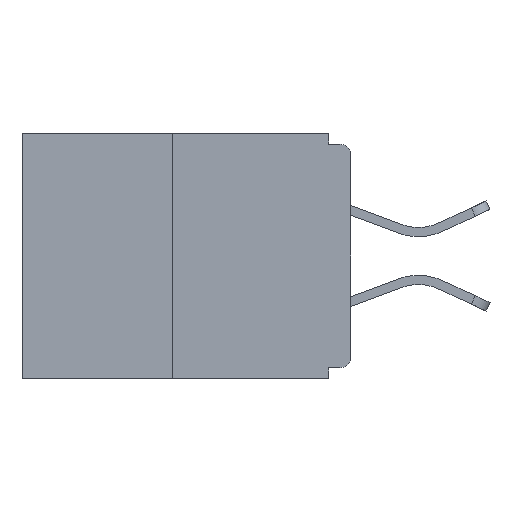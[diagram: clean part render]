
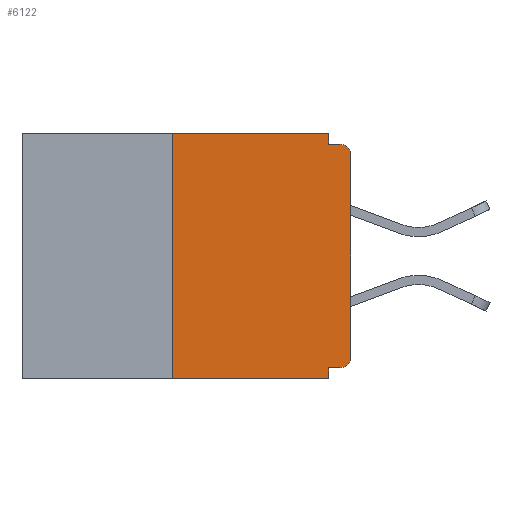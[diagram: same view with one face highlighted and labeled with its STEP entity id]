
A CAD part, left-side view. The second image highlights one B-rep face of the part: STEP entity #6122.
In plain terms, the highlighted planar face has unit normal (-1, 0, 0).
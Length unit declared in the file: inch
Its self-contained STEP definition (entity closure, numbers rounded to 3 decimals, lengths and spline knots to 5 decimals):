
#109 = CARTESIAN_POINT ( 'NONE',  ( 0., 0.015, -0.03 ) ) ;
#169 = ORIENTED_EDGE ( 'NONE', *, *, #7103, .T. ) ;
#346 = AXIS2_PLACEMENT_3D ( 'NONE', #14062, #10802, #5309 ) ;
#379 = VECTOR ( 'NONE', #10592, 39.37008 ) ;
#384 = EDGE_CURVE ( 'NONE', #3862, #9873, #11531, .T. ) ;
#671 = CARTESIAN_POINT ( 'NONE',  ( 0., 0.031, -0.343 ) ) ;
#859 = DIRECTION ( 'NONE',  ( 0., -1., 0. ) ) ;
#1123 = ORIENTED_EDGE ( 'NONE', *, *, #3468, .T. ) ;
#1216 = VERTEX_POINT ( 'NONE', #6062 ) ;
#1294 = CARTESIAN_POINT ( 'NONE',  ( 0., 0.46, -0.343 ) ) ;
#1317 = VERTEX_POINT ( 'NONE', #8545 ) ;
#1413 = VECTOR ( 'NONE', #2914, 39.37008 ) ;
#1504 = VERTEX_POINT ( 'NONE', #9048 ) ;
#2130 = ORIENTED_EDGE ( 'NONE', *, *, #5068, .F. ) ;
#2186 = CARTESIAN_POINT ( 'NONE',  ( 0., 0., -0.03 ) ) ;
#2205 = VERTEX_POINT ( 'NONE', #10170 ) ;
#2299 = CARTESIAN_POINT ( 'NONE',  ( 0., 0.031, 0. ) ) ;
#2351 = CARTESIAN_POINT ( 'NONE',  ( 0., 0.015, -0.015 ) ) ;
#2426 = LINE ( 'NONE', #5913, #7983 ) ;
#2914 = DIRECTION ( 'NONE',  ( 0., -1., 0. ) ) ;
#3018 = VERTEX_POINT ( 'NONE', #6176 ) ;
#3104 = CARTESIAN_POINT ( 'NONE',  ( 0., 0.46, 0. ) ) ;
#3373 = CARTESIAN_POINT ( 'NONE',  ( 0., 0.46, 0. ) ) ;
#3398 = DIRECTION ( 'NONE',  ( -1., 0., 0. ) ) ;
#3468 = EDGE_CURVE ( 'NONE', #1216, #13208, #2426, .T. ) ;
#3528 = VECTOR ( 'NONE', #7657, 39.37008 ) ;
#3664 = LINE ( 'NONE', #6067, #379 ) ;
#3862 = VERTEX_POINT ( 'NONE', #13517 ) ;
#3998 = DIRECTION ( 'NONE',  ( 0., 0., -1. ) ) ;
#4060 = ORIENTED_EDGE ( 'NONE', *, *, #7364, .T. ) ;
#4066 = ORIENTED_EDGE ( 'NONE', *, *, #5152, .F. ) ;
#4101 = CIRCLE ( 'NONE', #4241, 0.015 ) ;
#4130 = ORIENTED_EDGE ( 'NONE', *, *, #4430, .F. ) ;
#4160 = LINE ( 'NONE', #671, #8690 ) ;
#4241 = AXIS2_PLACEMENT_3D ( 'NONE', #109, #3398, #11175 ) ;
#4396 = DIRECTION ( 'NONE',  ( 1., 0., 0. ) ) ;
#4430 = EDGE_CURVE ( 'NONE', #1504, #2205, #3664, .T. ) ;
#5024 = ORIENTED_EDGE ( 'NONE', *, *, #384, .F. ) ;
#5068 = EDGE_CURVE ( 'NONE', #7882, #3018, #14091, .T. ) ;
#5152 = EDGE_CURVE ( 'NONE', #3018, #1317, #4160, .T. ) ;
#5309 = DIRECTION ( 'NONE',  ( 0., 0., -1. ) ) ;
#5508 = DIRECTION ( 'NONE',  ( 0., 0., -1. ) ) ;
#5756 = DIRECTION ( 'NONE',  ( 0., -1., 0. ) ) ;
#5913 = CARTESIAN_POINT ( 'NONE',  ( 0., 0., 0. ) ) ;
#6062 = CARTESIAN_POINT ( 'NONE',  ( 0., 0., -0.313 ) ) ;
#6067 = CARTESIAN_POINT ( 'NONE',  ( 0., 0.25, 0. ) ) ;
#6122 = ADVANCED_FACE ( 'NONE', ( #12318 ), #6695, .F. ) ;
#6176 = CARTESIAN_POINT ( 'NONE',  ( 0., 0.031, -0.328 ) ) ;
#6589 = CARTESIAN_POINT ( 'NONE',  ( 0., 0.015, -0.328 ) ) ;
#6695 = PLANE ( 'NONE',  #8813 ) ;
#7103 = EDGE_CURVE ( 'NONE', #7882, #1216, #7399, .T. ) ;
#7364 = EDGE_CURVE ( 'NONE', #13208, #9873, #4101, .T. ) ;
#7399 = CIRCLE ( 'NONE', #346, 0.015 ) ;
#7434 = CARTESIAN_POINT ( 'NONE',  ( 0., 0., -0.015 ) ) ;
#7574 = ORIENTED_EDGE ( 'NONE', *, *, #11496, .T. ) ;
#7657 = DIRECTION ( 'NONE',  ( 0., 0., -1. ) ) ;
#7812 = VECTOR ( 'NONE', #8400, 39.37008 ) ;
#7882 = VERTEX_POINT ( 'NONE', #6589 ) ;
#7983 = VECTOR ( 'NONE', #8113, 39.37008 ) ;
#7995 = VECTOR ( 'NONE', #5756, 39.37008 ) ;
#8113 = DIRECTION ( 'NONE',  ( 0., 0., 1. ) ) ;
#8400 = DIRECTION ( 'NONE',  ( 0., 1., 0. ) ) ;
#8540 = EDGE_CURVE ( 'NONE', #12053, #3862, #11366, .T. ) ;
#8545 = CARTESIAN_POINT ( 'NONE',  ( 0., 0.031, -0.343 ) ) ;
#8690 = VECTOR ( 'NONE', #3998, 39.37008 ) ;
#8813 = AXIS2_PLACEMENT_3D ( 'NONE', #3373, #4396, #5508 ) ;
#9048 = CARTESIAN_POINT ( 'NONE',  ( 0., 0.25, -0.343 ) ) ;
#9873 = VERTEX_POINT ( 'NONE', #2351 ) ;
#10170 = CARTESIAN_POINT ( 'NONE',  ( 0., 0.25, 0. ) ) ;
#10174 = ORIENTED_EDGE ( 'NONE', *, *, #8540, .F. ) ;
#10241 = EDGE_CURVE ( 'NONE', #2205, #12053, #11855, .T. ) ;
#10592 = DIRECTION ( 'NONE',  ( 0., 0., 1. ) ) ;
#10802 = DIRECTION ( 'NONE',  ( -1., 0., 0. ) ) ;
#10960 = LINE ( 'NONE', #1294, #7995 ) ;
#11175 = DIRECTION ( 'NONE',  ( 0., 0., -1. ) ) ;
#11192 = VECTOR ( 'NONE', #859, 39.37008 ) ;
#11366 = LINE ( 'NONE', #12291, #3528 ) ;
#11496 = EDGE_CURVE ( 'NONE', #1504, #1317, #10960, .T. ) ;
#11531 = LINE ( 'NONE', #7434, #11192 ) ;
#11855 = LINE ( 'NONE', #3104, #1413 ) ;
#12053 = VERTEX_POINT ( 'NONE', #2299 ) ;
#12291 = CARTESIAN_POINT ( 'NONE',  ( 0., 0.031, 0. ) ) ;
#12318 = FACE_OUTER_BOUND ( 'NONE', #13039, .T. ) ;
#12770 = CARTESIAN_POINT ( 'NONE',  ( 0., 0., -0.328 ) ) ;
#13039 = EDGE_LOOP ( 'NONE', ( #13160, #4130, #7574, #4066, #2130, #169, #1123, #4060, #5024, #10174 ) ) ;
#13160 = ORIENTED_EDGE ( 'NONE', *, *, #10241, .F. ) ;
#13208 = VERTEX_POINT ( 'NONE', #2186 ) ;
#13517 = CARTESIAN_POINT ( 'NONE',  ( 0., 0.031, -0.015 ) ) ;
#14062 = CARTESIAN_POINT ( 'NONE',  ( 0., 0.015, -0.313 ) ) ;
#14091 = LINE ( 'NONE', #12770, #7812 ) ;
